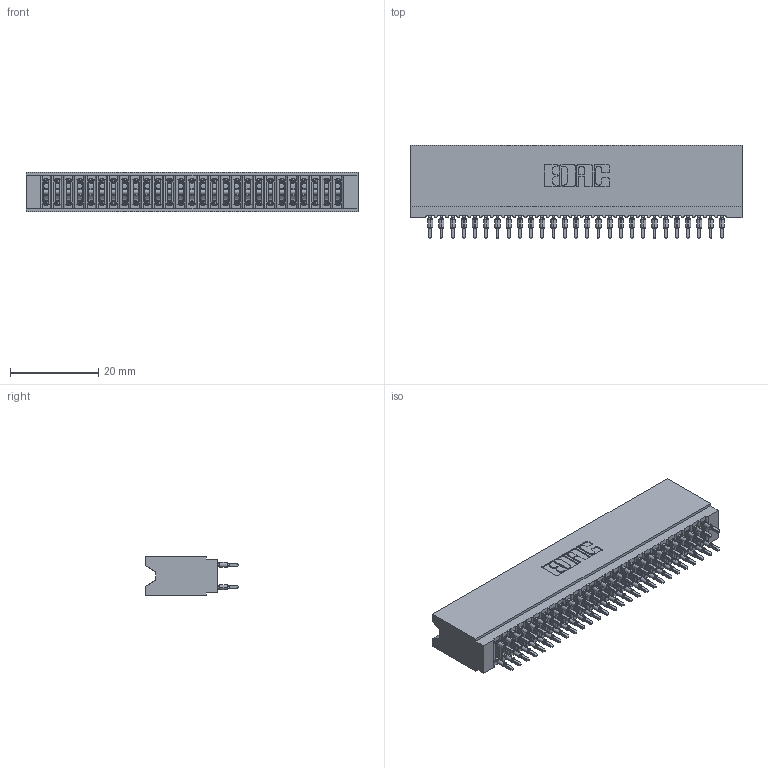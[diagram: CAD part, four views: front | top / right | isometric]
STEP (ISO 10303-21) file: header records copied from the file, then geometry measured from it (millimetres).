
FILE_DESCRIPTION (( 'STEP AP203' ), '1' );
FILE_NAME ('745-054-560-206.STEP', '2026-02-26T18:36:26', ( '' ), ( '' ), 'SwSTEP 2.0', 'SolidWorks 2023', '' );
FILE_SCHEMA (( 'CONFIG_CONTROL_DESIGN' ));
Length unit declared in the file: millimetre
Products named in the file (3): 745-054-560-206; 745 Part_Insulator Option - 06; 745-292-001_560
Assembly tree (55 placements, depth 2):
  745-054-560-206
    745 Part_Insulator Option - 06
    745-292-001_560  x54
Bounding box: 75.18 x 21.22 x 8.89 mm (x, y, z)
Volume: 7038.8 mm3; surface area: 14841 mm2
Topology: 55 solids, 55 shells, 5415 faces, 14813 edges, 9406 vertices
Faces by surface type: plane 2810, cylinder 1201, bspline 1080, torus 324
Entity records: 47846 total; most frequent: CARTESIAN_POINT 8808, ORIENTED_EDGE 8214, DIRECTION 7193, EDGE_CURVE 4107, VECTOR 3755, LINE 3755, VERTEX_POINT 2622, AXIS2_PLACEMENT_3D 1719
